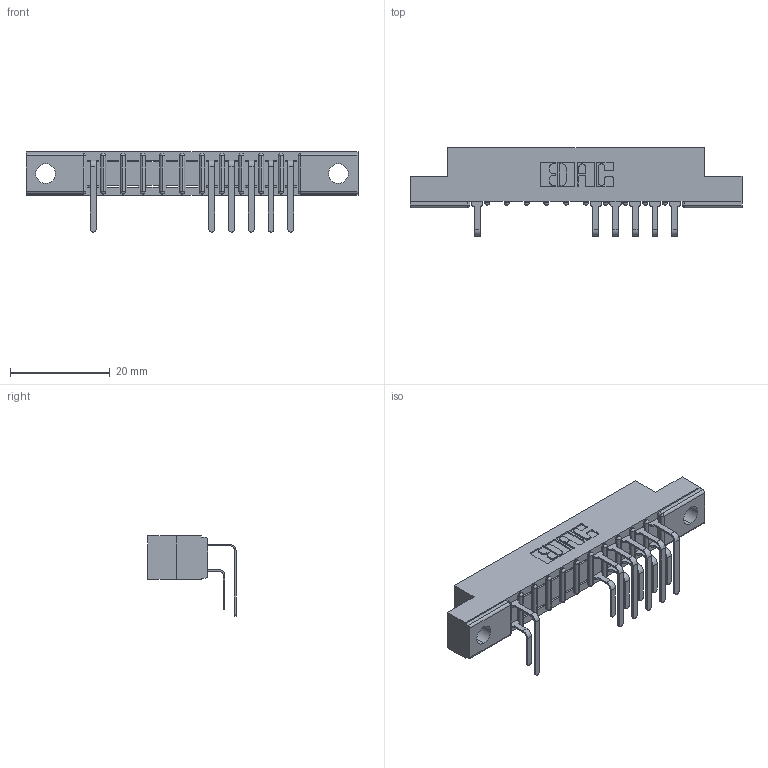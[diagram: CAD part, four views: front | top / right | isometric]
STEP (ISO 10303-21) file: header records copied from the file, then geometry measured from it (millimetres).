
FILE_DESCRIPTION (( 'STEP AP203' ), '1' );
FILE_NAME ('357-011-559-104.STEP', '2018-08-07T03:59:34', ( '' ), ( '' ), 'SwSTEP 2.0', 'SolidWorks 2016', '' );
FILE_SCHEMA (( 'CONFIG_CONTROL_DESIGN' ));
Length unit declared in the file: inch
Products named in the file (4): 307-290-001_559 - 2 (Single); 357-011-559-104; 307 Part_.156 Dia Mounting Holes; 307-290-001_558 559 - 1 (Single)
Assembly tree (13 placements, depth 2):
  357-011-559-104
    307 Part_.156 Dia Mounting Holes
    307-290-001_558 559 - 1 (Single)  x6
    307-290-001_559 - 2 (Single)  x6
Bounding box: 66.6 x 17.69 x 16.08 mm (x, y, z)
Volume: 4175.3 mm3; surface area: 6224.3 mm2
Topology: 13 solids, 13 shells, 844 faces, 2383 edges, 1538 vertices
Faces by surface type: plane 540, cylinder 280, sphere 24
Entity records: 15149 total; most frequent: CARTESIAN_POINT 2537, ORIENTED_EDGE 2518, DIRECTION 2479, EDGE_CURVE 1259, LINE 959, VECTOR 959, VERTEX_POINT 818, AXIS2_PLACEMENT_3D 760
